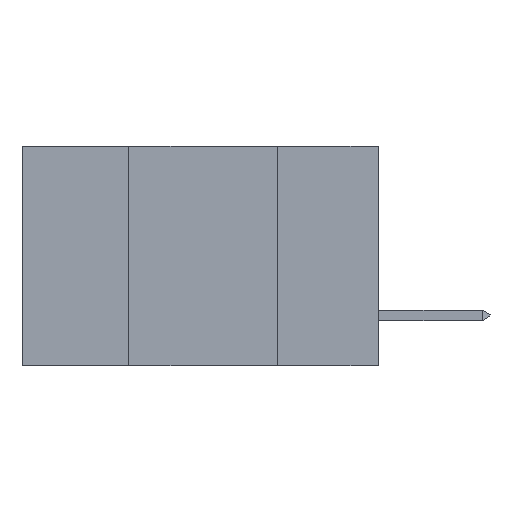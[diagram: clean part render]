
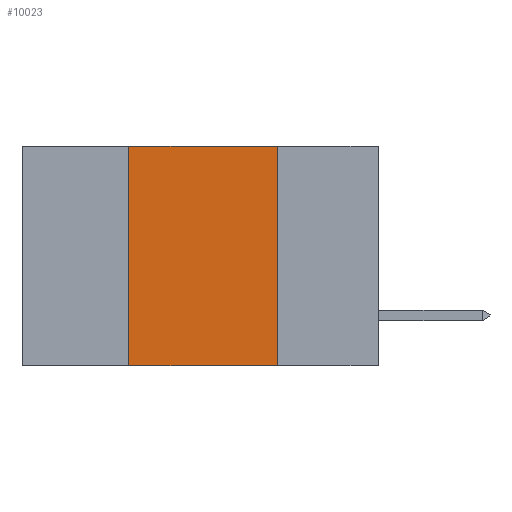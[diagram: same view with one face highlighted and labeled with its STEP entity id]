
A CAD part, left-side view. The second image highlights one B-rep face of the part: STEP entity #10023.
In plain terms, the highlighted planar face has unit normal (-1, 0, 0).
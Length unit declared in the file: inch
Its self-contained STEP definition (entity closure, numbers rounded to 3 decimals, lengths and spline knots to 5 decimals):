
#69 = VECTOR ( 'NONE', #6583, 39.37008 ) ;
#1473 = VECTOR ( 'NONE', #13344, 39.37008 ) ;
#1650 = FACE_OUTER_BOUND ( 'NONE', #21995, .T. ) ;
#2000 = CARTESIAN_POINT ( 'NONE',  ( 0., 0.6, 0. ) ) ;
#2490 = ORIENTED_EDGE ( 'NONE', *, *, #9329, .F. ) ;
#2939 = CARTESIAN_POINT ( 'NONE',  ( 0., 0.6, -0.37 ) ) ;
#3514 = CARTESIAN_POINT ( 'NONE',  ( 0., 0.17, -0.37 ) ) ;
#3566 = CARTESIAN_POINT ( 'NONE',  ( 0., 0.17, -0.37 ) ) ;
#5121 = VERTEX_POINT ( 'NONE', #16522 ) ;
#5584 = EDGE_CURVE ( 'NONE', #19477, #15247, #13041, .T. ) ;
#6583 = DIRECTION ( 'NONE',  ( 0., 0., 1. ) ) ;
#7422 = AXIS2_PLACEMENT_3D ( 'NONE', #2000, #14766, #19003 ) ;
#9329 = EDGE_CURVE ( 'NONE', #5121, #19477, #9354, .T. ) ;
#9354 = LINE ( 'NONE', #20848, #1473 ) ;
#10023 = ADVANCED_FACE ( 'NONE', ( #1650 ), #16910, .F. ) ;
#13041 = LINE ( 'NONE', #3566, #24135 ) ;
#13344 = DIRECTION ( 'NONE',  ( 0., -1., 0. ) ) ;
#13880 = CARTESIAN_POINT ( 'NONE',  ( 0., 0.17, 0. ) ) ;
#14272 = LINE ( 'NONE', #2939, #20456 ) ;
#14766 = DIRECTION ( 'NONE',  ( 1., 0., 0. ) ) ;
#15247 = VERTEX_POINT ( 'NONE', #3514 ) ;
#15638 = ORIENTED_EDGE ( 'NONE', *, *, #5584, .F. ) ;
#16049 = CARTESIAN_POINT ( 'NONE',  ( 0., 0.42, -0.37 ) ) ;
#16406 = ORIENTED_EDGE ( 'NONE', *, *, #17165, .F. ) ;
#16522 = CARTESIAN_POINT ( 'NONE',  ( 0., 0.42, 0. ) ) ;
#16910 = PLANE ( 'NONE',  #7422 ) ;
#17165 = EDGE_CURVE ( 'NONE', #18606, #5121, #23589, .T. ) ;
#18189 = DIRECTION ( 'NONE',  ( 0., -1., 0. ) ) ;
#18606 = VERTEX_POINT ( 'NONE', #21794 ) ;
#19003 = DIRECTION ( 'NONE',  ( 0., 0., -1. ) ) ;
#19477 = VERTEX_POINT ( 'NONE', #13880 ) ;
#19872 = ORIENTED_EDGE ( 'NONE', *, *, #20061, .T. ) ;
#20061 = EDGE_CURVE ( 'NONE', #18606, #15247, #14272, .T. ) ;
#20456 = VECTOR ( 'NONE', #18189, 39.37008 ) ;
#20848 = CARTESIAN_POINT ( 'NONE',  ( 0., 0.6, 0. ) ) ;
#21794 = CARTESIAN_POINT ( 'NONE',  ( 0., 0.42, -0.37 ) ) ;
#21995 = EDGE_LOOP ( 'NONE', ( #15638, #2490, #16406, #19872 ) ) ;
#23589 = LINE ( 'NONE', #16049, #69 ) ;
#24135 = VECTOR ( 'NONE', #24715, 39.37008 ) ;
#24715 = DIRECTION ( 'NONE',  ( 0., 0., -1. ) ) ;
